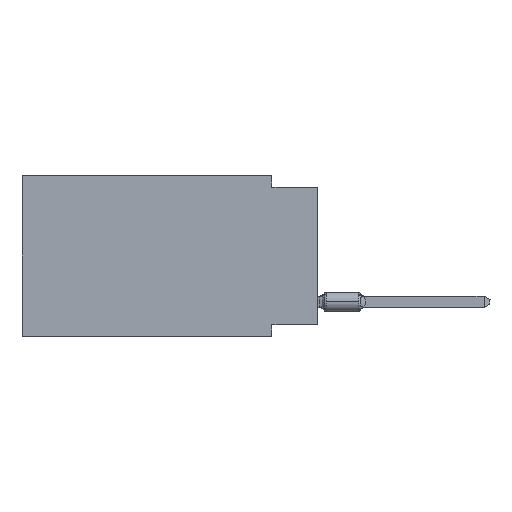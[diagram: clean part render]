
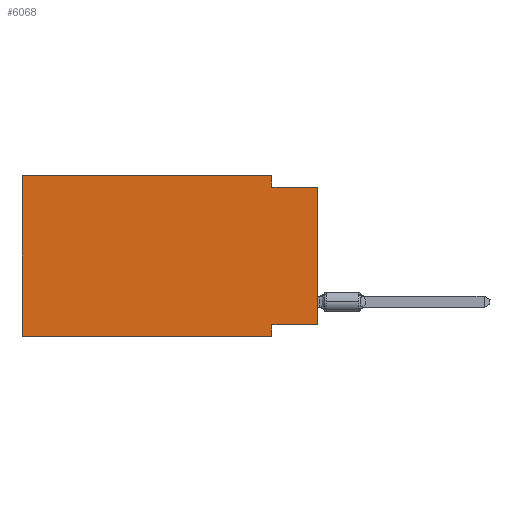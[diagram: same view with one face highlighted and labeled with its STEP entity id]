
A CAD part, left-side view. The second image highlights one B-rep face of the part: STEP entity #6068.
In plain terms, the highlighted planar face has unit normal (-1, 0, 0).
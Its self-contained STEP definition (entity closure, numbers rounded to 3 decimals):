
#1471 = VECTOR ( 'NONE', #8087, 1000. ) ;
#3535 = CARTESIAN_POINT ( 'NONE',  ( 0., 0., -0.635 ) ) ;
#3694 = EDGE_CURVE ( 'NONE', #68717, #73568, #79223, .T. ) ;
#4737 = ORIENTED_EDGE ( 'NONE', *, *, #40029, .F. ) ;
#5775 = CARTESIAN_POINT ( 'NONE',  ( 0., 2.54, -8.255 ) ) ;
#6068 = ADVANCED_FACE ( 'NONE', ( #37404 ), #76013, .F. ) ;
#6352 = CARTESIAN_POINT ( 'NONE',  ( 0., 16.383, 0. ) ) ;
#7043 = VECTOR ( 'NONE', #33857, 1000. ) ;
#8087 = DIRECTION ( 'NONE',  ( 0., 0., -1. ) ) ;
#12628 = DIRECTION ( 'NONE',  ( 0., 0., -1. ) ) ;
#14643 = EDGE_CURVE ( 'NONE', #54504, #75008, #82211, .T. ) ;
#17464 = CARTESIAN_POINT ( 'NONE',  ( 0., 16.383, 0. ) ) ;
#18575 = DIRECTION ( 'NONE',  ( 0., -1., 0. ) ) ;
#19170 = ORIENTED_EDGE ( 'NONE', *, *, #14643, .T. ) ;
#20602 = EDGE_CURVE ( 'NONE', #68717, #55652, #45217, .T. ) ;
#21723 = CARTESIAN_POINT ( 'NONE',  ( 0., 0., 0. ) ) ;
#24035 = LINE ( 'NONE', #25287, #24568 ) ;
#24269 = CARTESIAN_POINT ( 'NONE',  ( 0., 2.54, -8.89 ) ) ;
#24479 = CARTESIAN_POINT ( 'NONE',  ( 0., 16.383, 0. ) ) ;
#24568 = VECTOR ( 'NONE', #76059, 1000. ) ;
#24712 = DIRECTION ( 'NONE',  ( 0., -1., 0. ) ) ;
#25287 = CARTESIAN_POINT ( 'NONE',  ( 0., 0., -0.635 ) ) ;
#28212 = CARTESIAN_POINT ( 'NONE',  ( 0., 2.54, 0. ) ) ;
#30301 = EDGE_CURVE ( 'NONE', #71068, #69850, #33675, .T. ) ;
#31056 = AXIS2_PLACEMENT_3D ( 'NONE', #6352, #76429, #12628 ) ;
#32012 = ORIENTED_EDGE ( 'NONE', *, *, #30301, .F. ) ;
#33675 = LINE ( 'NONE', #28212, #1471 ) ;
#33857 = DIRECTION ( 'NONE',  ( 0., 1., 0. ) ) ;
#34735 = EDGE_CURVE ( 'NONE', #54504, #69981, #59869, .T. ) ;
#35990 = ORIENTED_EDGE ( 'NONE', *, *, #34735, .F. ) ;
#36213 = CARTESIAN_POINT ( 'NONE',  ( 0., 0., -8.255 ) ) ;
#36889 = VECTOR ( 'NONE', #51788, 1000. ) ;
#37373 = ORIENTED_EDGE ( 'NONE', *, *, #20602, .F. ) ;
#37404 = FACE_OUTER_BOUND ( 'NONE', #40926, .T. ) ;
#40029 = EDGE_CURVE ( 'NONE', #69850, #73568, #24035, .T. ) ;
#40926 = EDGE_LOOP ( 'NONE', ( #49513, #4737, #32012, #58386, #35990, #19170, #50251, #37373 ) ) ;
#45217 = LINE ( 'NONE', #65740, #7043 ) ;
#46979 = EDGE_CURVE ( 'NONE', #55652, #75008, #51378, .T. ) ;
#49513 = ORIENTED_EDGE ( 'NONE', *, *, #3694, .T. ) ;
#49663 = CARTESIAN_POINT ( 'NONE',  ( 0., 2.54, -0.635 ) ) ;
#50251 = ORIENTED_EDGE ( 'NONE', *, *, #46979, .F. ) ;
#50737 = CARTESIAN_POINT ( 'NONE',  ( 0., 16.383, -8.89 ) ) ;
#51378 = LINE ( 'NONE', #70253, #36889 ) ;
#51788 = DIRECTION ( 'NONE',  ( 0., 0., -1. ) ) ;
#54504 = VERTEX_POINT ( 'NONE', #67826 ) ;
#55652 = VERTEX_POINT ( 'NONE', #5775 ) ;
#58386 = ORIENTED_EDGE ( 'NONE', *, *, #78935, .F. ) ;
#59530 = VECTOR ( 'NONE', #72908, 1000. ) ;
#59869 = LINE ( 'NONE', #17464, #65171 ) ;
#63468 = CARTESIAN_POINT ( 'NONE',  ( 0., 16.383, 0. ) ) ;
#65171 = VECTOR ( 'NONE', #82096, 1000. ) ;
#65740 = CARTESIAN_POINT ( 'NONE',  ( 0., 0., -8.255 ) ) ;
#67826 = CARTESIAN_POINT ( 'NONE',  ( 0., 16.383, -8.89 ) ) ;
#68717 = VERTEX_POINT ( 'NONE', #36213 ) ;
#69850 = VERTEX_POINT ( 'NONE', #49663 ) ;
#69981 = VERTEX_POINT ( 'NONE', #24479 ) ;
#70253 = CARTESIAN_POINT ( 'NONE',  ( 0., 2.54, -8.89 ) ) ;
#71068 = VERTEX_POINT ( 'NONE', #82467 ) ;
#72908 = DIRECTION ( 'NONE',  ( 0., 0., 1. ) ) ;
#73568 = VERTEX_POINT ( 'NONE', #3535 ) ;
#75008 = VERTEX_POINT ( 'NONE', #24269 ) ;
#76013 = PLANE ( 'NONE',  #31056 ) ;
#76059 = DIRECTION ( 'NONE',  ( 0., -1., 0. ) ) ;
#76065 = LINE ( 'NONE', #63468, #82355 ) ;
#76429 = DIRECTION ( 'NONE',  ( 1., 0., 0. ) ) ;
#78935 = EDGE_CURVE ( 'NONE', #69981, #71068, #76065, .T. ) ;
#79223 = LINE ( 'NONE', #21723, #59530 ) ;
#80740 = VECTOR ( 'NONE', #24712, 1000. ) ;
#82096 = DIRECTION ( 'NONE',  ( 0., 0., 1. ) ) ;
#82211 = LINE ( 'NONE', #50737, #80740 ) ;
#82355 = VECTOR ( 'NONE', #18575, 1000. ) ;
#82467 = CARTESIAN_POINT ( 'NONE',  ( 0., 2.54, 0. ) ) ;
